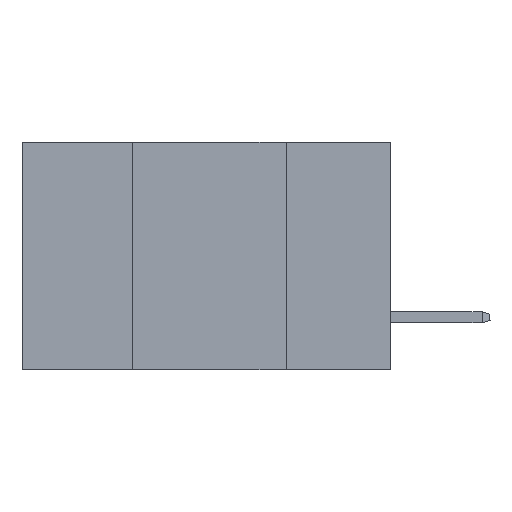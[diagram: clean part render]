
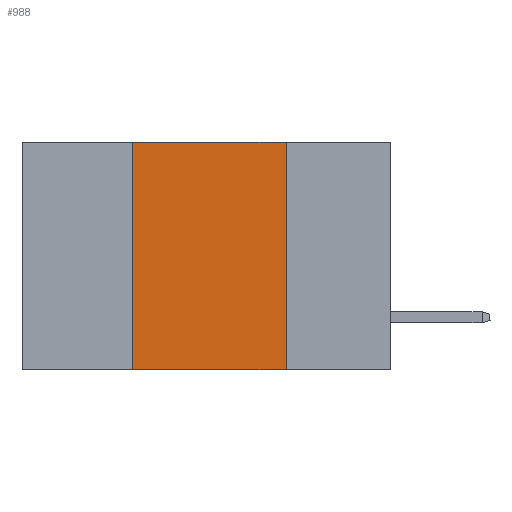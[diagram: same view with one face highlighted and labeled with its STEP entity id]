
A CAD part, left-side view. The second image highlights one B-rep face of the part: STEP entity #988.
In plain terms, the highlighted planar face has unit normal (-1, 0, 0).
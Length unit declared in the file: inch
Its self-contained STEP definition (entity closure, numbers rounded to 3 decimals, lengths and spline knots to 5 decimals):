
#87 = VERTEX_POINT ( 'NONE', #9852 ) ;
#954 = EDGE_CURVE ( 'NONE', #6097, #3371, #5004, .T. ) ;
#988 = ADVANCED_FACE ( 'NONE', ( #9868 ), #4798, .F. ) ;
#1430 = AXIS2_PLACEMENT_3D ( 'NONE', #12342, #7821, #10951 ) ;
#1500 = DIRECTION ( 'NONE',  ( 0., 0., -1. ) ) ;
#2193 = DIRECTION ( 'NONE',  ( 0., 0., 1. ) ) ;
#2339 = EDGE_LOOP ( 'NONE', ( #12893, #2632, #9907, #15042 ) ) ;
#2632 = ORIENTED_EDGE ( 'NONE', *, *, #13259, .F. ) ;
#3371 = VERTEX_POINT ( 'NONE', #10085 ) ;
#4539 = EDGE_CURVE ( 'NONE', #87, #3371, #11187, .T. ) ;
#4798 = PLANE ( 'NONE',  #1430 ) ;
#5004 = LINE ( 'NONE', #9263, #12012 ) ;
#5195 = LINE ( 'NONE', #16125, #14131 ) ;
#6061 = CARTESIAN_POINT ( 'NONE',  ( 0., 0.42, 0. ) ) ;
#6097 = VERTEX_POINT ( 'NONE', #6776 ) ;
#6776 = CARTESIAN_POINT ( 'NONE',  ( 0., 0.42, -0.37 ) ) ;
#7666 = CARTESIAN_POINT ( 'NONE',  ( 0., 0.17, 0. ) ) ;
#7821 = DIRECTION ( 'NONE',  ( 1., 0., 0. ) ) ;
#9263 = CARTESIAN_POINT ( 'NONE',  ( 0., 0.6, -0.37 ) ) ;
#9852 = CARTESIAN_POINT ( 'NONE',  ( 0., 0.17, 0. ) ) ;
#9868 = FACE_OUTER_BOUND ( 'NONE', #2339, .T. ) ;
#9907 = ORIENTED_EDGE ( 'NONE', *, *, #19993, .F. ) ;
#9999 = VERTEX_POINT ( 'NONE', #6061 ) ;
#10085 = CARTESIAN_POINT ( 'NONE',  ( 0., 0.17, -0.37 ) ) ;
#10951 = DIRECTION ( 'NONE',  ( 0., 0., -1. ) ) ;
#11187 = LINE ( 'NONE', #7666, #18445 ) ;
#11631 = CARTESIAN_POINT ( 'NONE',  ( 0., 0.6, 0. ) ) ;
#12012 = VECTOR ( 'NONE', #12408, 39.37008 ) ;
#12342 = CARTESIAN_POINT ( 'NONE',  ( 0., 0.6, 0. ) ) ;
#12408 = DIRECTION ( 'NONE',  ( 0., -1., 0. ) ) ;
#12893 = ORIENTED_EDGE ( 'NONE', *, *, #4539, .F. ) ;
#13259 = EDGE_CURVE ( 'NONE', #9999, #87, #19896, .T. ) ;
#14131 = VECTOR ( 'NONE', #2193, 39.37008 ) ;
#15042 = ORIENTED_EDGE ( 'NONE', *, *, #954, .T. ) ;
#16125 = CARTESIAN_POINT ( 'NONE',  ( 0., 0.42, 0. ) ) ;
#18445 = VECTOR ( 'NONE', #1500, 39.37008 ) ;
#19239 = DIRECTION ( 'NONE',  ( 0., -1., 0. ) ) ;
#19411 = VECTOR ( 'NONE', #19239, 39.37008 ) ;
#19896 = LINE ( 'NONE', #11631, #19411 ) ;
#19993 = EDGE_CURVE ( 'NONE', #6097, #9999, #5195, .T. ) ;
